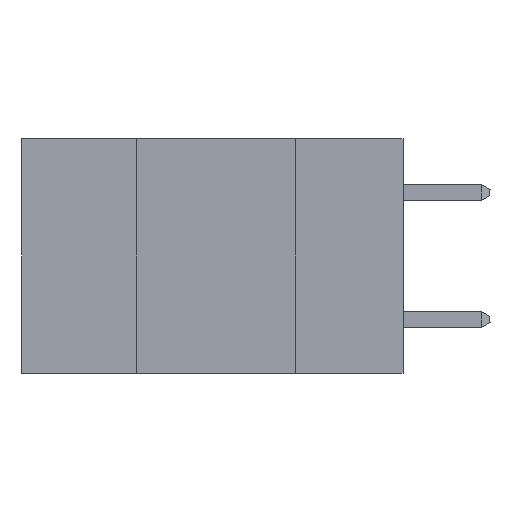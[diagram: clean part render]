
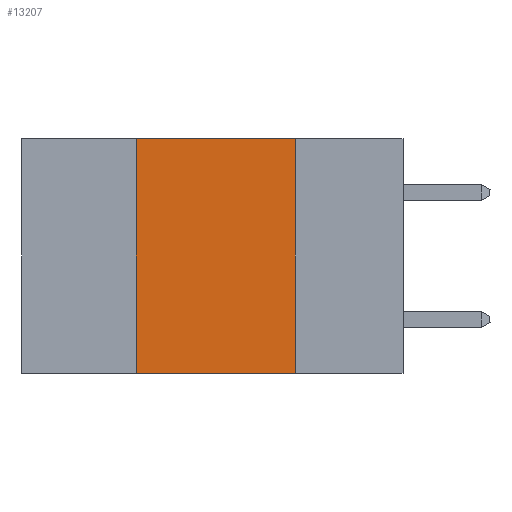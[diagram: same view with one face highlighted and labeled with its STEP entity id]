
A CAD part, left-side view. The second image highlights one B-rep face of the part: STEP entity #13207.
In plain terms, the highlighted planar face has unit normal (-1, 0, 0).
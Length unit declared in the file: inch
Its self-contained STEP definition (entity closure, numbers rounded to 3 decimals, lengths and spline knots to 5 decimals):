
#44 = AXIS2_PLACEMENT_3D ( 'NONE', #20704, #13917, #3255 ) ;
#2501 = LINE ( 'NONE', #19576, #11482 ) ;
#3122 = VERTEX_POINT ( 'NONE', #9455 ) ;
#3255 = DIRECTION ( 'NONE',  ( 0., 0., -1. ) ) ;
#3401 = LINE ( 'NONE', #17674, #12354 ) ;
#3670 = VECTOR ( 'NONE', #9517, 39.37008 ) ;
#4811 = EDGE_CURVE ( 'NONE', #13966, #17483, #13166, .T. ) ;
#5001 = PLANE ( 'NONE',  #44 ) ;
#6476 = EDGE_CURVE ( 'NONE', #7418, #13966, #2501, .T. ) ;
#6514 = LINE ( 'NONE', #17061, #16423 ) ;
#6567 = DIRECTION ( 'NONE',  ( 0., 0., 1. ) ) ;
#7418 = VERTEX_POINT ( 'NONE', #7747 ) ;
#7747 = CARTESIAN_POINT ( 'NONE',  ( 0., 0.42, 0. ) ) ;
#8607 = CARTESIAN_POINT ( 'NONE',  ( 0., 0.17, 0. ) ) ;
#9455 = CARTESIAN_POINT ( 'NONE',  ( 0., 0.42, -0.37 ) ) ;
#9517 = DIRECTION ( 'NONE',  ( 0., 0., -1. ) ) ;
#11160 = CARTESIAN_POINT ( 'NONE',  ( 0., 0.17, 0. ) ) ;
#11482 = VECTOR ( 'NONE', #19773, 39.37008 ) ;
#12114 = ORIENTED_EDGE ( 'NONE', *, *, #19295, .T. ) ;
#12354 = VECTOR ( 'NONE', #19399, 39.37008 ) ;
#13166 = LINE ( 'NONE', #8607, #3670 ) ;
#13207 = ADVANCED_FACE ( 'NONE', ( #22285 ), #5001, .F. ) ;
#13917 = DIRECTION ( 'NONE',  ( 1., 0., 0. ) ) ;
#13966 = VERTEX_POINT ( 'NONE', #11160 ) ;
#14554 = ORIENTED_EDGE ( 'NONE', *, *, #22692, .F. ) ;
#16423 = VECTOR ( 'NONE', #6567, 39.37008 ) ;
#17061 = CARTESIAN_POINT ( 'NONE',  ( 0., 0.42, 0. ) ) ;
#17483 = VERTEX_POINT ( 'NONE', #19540 ) ;
#17674 = CARTESIAN_POINT ( 'NONE',  ( 0., 0.6, -0.37 ) ) ;
#18753 = ORIENTED_EDGE ( 'NONE', *, *, #4811, .F. ) ;
#19295 = EDGE_CURVE ( 'NONE', #3122, #17483, #3401, .T. ) ;
#19399 = DIRECTION ( 'NONE',  ( 0., -1., 0. ) ) ;
#19540 = CARTESIAN_POINT ( 'NONE',  ( 0., 0.17, -0.37 ) ) ;
#19576 = CARTESIAN_POINT ( 'NONE',  ( 0., 0.6, 0. ) ) ;
#19773 = DIRECTION ( 'NONE',  ( 0., -1., 0. ) ) ;
#20250 = EDGE_LOOP ( 'NONE', ( #18753, #20359, #14554, #12114 ) ) ;
#20359 = ORIENTED_EDGE ( 'NONE', *, *, #6476, .F. ) ;
#20704 = CARTESIAN_POINT ( 'NONE',  ( 0., 0.6, 0. ) ) ;
#22285 = FACE_OUTER_BOUND ( 'NONE', #20250, .T. ) ;
#22692 = EDGE_CURVE ( 'NONE', #3122, #7418, #6514, .T. ) ;
